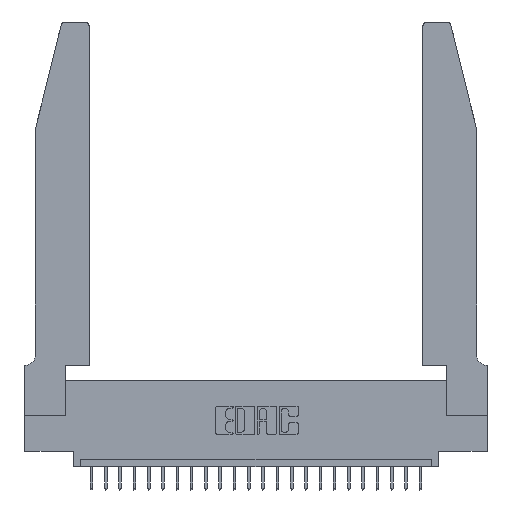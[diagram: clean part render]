
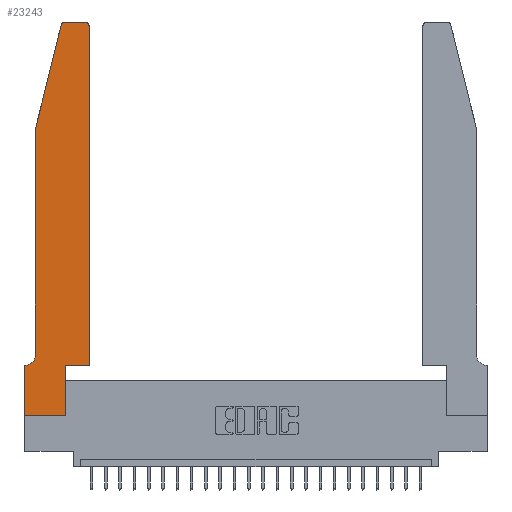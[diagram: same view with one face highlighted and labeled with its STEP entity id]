
A CAD part, top view. The second image highlights one B-rep face of the part: STEP entity #23243.
In plain terms, the highlighted planar face has unit normal (0, 0, 1).
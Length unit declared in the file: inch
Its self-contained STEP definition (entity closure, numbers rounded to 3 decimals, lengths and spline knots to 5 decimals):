
#17 = VERTEX_POINT ( 'NONE', #1038 ) ;
#164 = CARTESIAN_POINT ( 'NONE',  ( 0., 0.35, 0.37 ) ) ;
#499 = VERTEX_POINT ( 'NONE', #9481 ) ;
#1038 = CARTESIAN_POINT ( 'NONE',  ( 0., 0.35, 0.37 ) ) ;
#1136 = CIRCLE ( 'NONE', #16372, 0.03 ) ;
#1219 = DIRECTION ( 'NONE',  ( 1., 0., 0. ) ) ;
#1333 = ORIENTED_EDGE ( 'NONE', *, *, #2403, .T. ) ;
#1780 = EDGE_CURVE ( 'NONE', #19291, #17657, #18581, .T. ) ;
#1923 = VECTOR ( 'NONE', #10608, 39.37008 ) ;
#2403 = EDGE_CURVE ( 'NONE', #499, #18775, #5967, .T. ) ;
#2966 = EDGE_CURVE ( 'NONE', #12963, #6770, #20093, .T. ) ;
#3355 = DIRECTION ( 'NONE',  ( 0., 1., 0. ) ) ;
#3795 = CARTESIAN_POINT ( 'NONE',  ( 0.4205, 2.72, 0.37 ) ) ;
#3904 = DIRECTION ( 'NONE',  ( 0., 0., 1. ) ) ;
#4003 = CARTESIAN_POINT ( 'NONE',  ( 0.2865, 0.35, 0.37 ) ) ;
#4143 = ORIENTED_EDGE ( 'NONE', *, *, #11249, .T. ) ;
#4719 = ORIENTED_EDGE ( 'NONE', *, *, #18608, .T. ) ;
#4771 = EDGE_CURVE ( 'NONE', #24978, #9775, #20688, .T. ) ;
#4891 = DIRECTION ( 'NONE',  ( 0., -1., 0. ) ) ;
#5760 = CARTESIAN_POINT ( 'NONE',  ( 0.0755, 2., 0.37 ) ) ;
#5800 = ORIENTED_EDGE ( 'NONE', *, *, #8507, .T. ) ;
#5967 = LINE ( 'NONE', #8858, #24112 ) ;
#6113 = VECTOR ( 'NONE', #22655, 39.37008 ) ;
#6178 = PLANE ( 'NONE',  #9769 ) ;
#6311 = DIRECTION ( 'NONE',  ( 0., 1., 0. ) ) ;
#6721 = LINE ( 'NONE', #14429, #15346 ) ;
#6731 = EDGE_CURVE ( 'NONE', #17, #19291, #6721, .T. ) ;
#6770 = VERTEX_POINT ( 'NONE', #14850 ) ;
#6901 = CIRCLE ( 'NONE', #9035, 0.03 ) ;
#7571 = DIRECTION ( 'NONE',  ( 1., 0., 0. ) ) ;
#8059 = DIRECTION ( 'NONE',  ( 1., 0., 0. ) ) ;
#8093 = ORIENTED_EDGE ( 'NONE', *, *, #2966, .T. ) ;
#8507 = EDGE_CURVE ( 'NONE', #18775, #20206, #1136, .T. ) ;
#8521 = DIRECTION ( 'NONE',  ( 0., 0., -1. ) ) ;
#8858 = CARTESIAN_POINT ( 'NONE',  ( 0.2605, 2.75, 0.37 ) ) ;
#9035 = AXIS2_PLACEMENT_3D ( 'NONE', #3795, #17533, #7571 ) ;
#9481 = CARTESIAN_POINT ( 'NONE',  ( 0.4205, 2.75, 0.37 ) ) ;
#9558 = CARTESIAN_POINT ( 'NONE',  ( 0.284, 2.75, 0.37 ) ) ;
#9697 = CARTESIAN_POINT ( 'NONE',  ( 0.0055, 0.35, 0.37 ) ) ;
#9769 = AXIS2_PLACEMENT_3D ( 'NONE', #164, #17849, #8059 ) ;
#9775 = VERTEX_POINT ( 'NONE', #10046 ) ;
#10046 = CARTESIAN_POINT ( 'NONE',  ( 0.0755, 0.42, 0.37 ) ) ;
#10608 = DIRECTION ( 'NONE',  ( 0., -1., 0. ) ) ;
#11009 = AXIS2_PLACEMENT_3D ( 'NONE', #12983, #8521, #24862 ) ;
#11036 = ORIENTED_EDGE ( 'NONE', *, *, #1780, .T. ) ;
#11249 = EDGE_CURVE ( 'NONE', #23093, #17, #13479, .T. ) ;
#11271 = CARTESIAN_POINT ( 'NONE',  ( 0.0755, 2., 0.37 ) ) ;
#12072 = CARTESIAN_POINT ( 'NONE',  ( 0.0755, 2., 0.37 ) ) ;
#12230 = CARTESIAN_POINT ( 'NONE',  ( 0.2865, 0.35, 0.37 ) ) ;
#12297 = DIRECTION ( 'NONE',  ( 1., 0., 0. ) ) ;
#12811 = EDGE_CURVE ( 'NONE', #20206, #24978, #21098, .T. ) ;
#12849 = LINE ( 'NONE', #24775, #17482 ) ;
#12963 = VERTEX_POINT ( 'NONE', #17188 ) ;
#12983 = CARTESIAN_POINT ( 'NONE',  ( 0.0055, 0.42, 0.37 ) ) ;
#13020 = EDGE_CURVE ( 'NONE', #6770, #499, #6901, .T. ) ;
#13479 = LINE ( 'NONE', #20775, #6113 ) ;
#14429 = CARTESIAN_POINT ( 'NONE',  ( 0., 0., 0.37 ) ) ;
#14733 = ORIENTED_EDGE ( 'NONE', *, *, #18575, .T. ) ;
#14850 = CARTESIAN_POINT ( 'NONE',  ( 0.4505, 2.72, 0.37 ) ) ;
#14874 = VECTOR ( 'NONE', #3355, 39.37008 ) ;
#15112 = CARTESIAN_POINT ( 'NONE',  ( 0.4505, 0.35, 0.37 ) ) ;
#15346 = VECTOR ( 'NONE', #4891, 39.37008 ) ;
#15596 = CARTESIAN_POINT ( 'NONE',  ( 0.25487, 2.72718, 0.37 ) ) ;
#15671 = CARTESIAN_POINT ( 'NONE',  ( 0.284, 2.72, 0.37 ) ) ;
#16302 = FACE_OUTER_BOUND ( 'NONE', #22569, .T. ) ;
#16372 = AXIS2_PLACEMENT_3D ( 'NONE', #15671, #3904, #12297 ) ;
#17188 = CARTESIAN_POINT ( 'NONE',  ( 0.4505, 0.35, 0.37 ) ) ;
#17377 = VECTOR ( 'NONE', #19558, 39.37008 ) ;
#17482 = VECTOR ( 'NONE', #1219, 39.37008 ) ;
#17533 = DIRECTION ( 'NONE',  ( 0., 0., 1. ) ) ;
#17572 = CARTESIAN_POINT ( 'NONE',  ( 0., 0., 0.37 ) ) ;
#17657 = VERTEX_POINT ( 'NONE', #17917 ) ;
#17849 = DIRECTION ( 'NONE',  ( 0., 0., 1. ) ) ;
#17917 = CARTESIAN_POINT ( 'NONE',  ( 0.2865, 0., 0.37 ) ) ;
#18238 = DIRECTION ( 'NONE',  ( -0.239, -0.971, 0. ) ) ;
#18575 = EDGE_CURVE ( 'NONE', #9775, #23093, #22707, .T. ) ;
#18581 = LINE ( 'NONE', #17572, #17377 ) ;
#18608 = EDGE_CURVE ( 'NONE', #23737, #12963, #12849, .T. ) ;
#18775 = VERTEX_POINT ( 'NONE', #9558 ) ;
#19291 = VERTEX_POINT ( 'NONE', #23521 ) ;
#19558 = DIRECTION ( 'NONE',  ( 1., 0., 0. ) ) ;
#20093 = LINE ( 'NONE', #15112, #14874 ) ;
#20206 = VERTEX_POINT ( 'NONE', #15596 ) ;
#20315 = EDGE_CURVE ( 'NONE', #17657, #23737, #22605, .T. ) ;
#20688 = LINE ( 'NONE', #12072, #1923 ) ;
#20775 = CARTESIAN_POINT ( 'NONE',  ( 0.0755, 0.35, 0.37 ) ) ;
#20993 = ORIENTED_EDGE ( 'NONE', *, *, #12811, .T. ) ;
#21098 = LINE ( 'NONE', #11271, #23557 ) ;
#21930 = ORIENTED_EDGE ( 'NONE', *, *, #4771, .T. ) ;
#22522 = ORIENTED_EDGE ( 'NONE', *, *, #6731, .T. ) ;
#22569 = EDGE_LOOP ( 'NONE', ( #1333, #5800, #20993, #21930, #14733, #4143, #22522, #11036, #24105, #4719, #8093, #23311 ) ) ;
#22581 = VECTOR ( 'NONE', #6311, 39.37008 ) ;
#22605 = LINE ( 'NONE', #12230, #22581 ) ;
#22655 = DIRECTION ( 'NONE',  ( -1., 0., 0. ) ) ;
#22707 = CIRCLE ( 'NONE', #11009, 0.07 ) ;
#23093 = VERTEX_POINT ( 'NONE', #9697 ) ;
#23243 = ADVANCED_FACE ( 'NONE', ( #16302 ), #6178, .T. ) ;
#23311 = ORIENTED_EDGE ( 'NONE', *, *, #13020, .T. ) ;
#23521 = CARTESIAN_POINT ( 'NONE',  ( 0., 0., 0.37 ) ) ;
#23557 = VECTOR ( 'NONE', #18238, 39.37008 ) ;
#23737 = VERTEX_POINT ( 'NONE', #4003 ) ;
#24105 = ORIENTED_EDGE ( 'NONE', *, *, #20315, .T. ) ;
#24112 = VECTOR ( 'NONE', #24184, 39.37008 ) ;
#24184 = DIRECTION ( 'NONE',  ( -1., 0., 0. ) ) ;
#24775 = CARTESIAN_POINT ( 'NONE',  ( 0.4505, 0.35, 0.37 ) ) ;
#24862 = DIRECTION ( 'NONE',  ( -1., 0., 0. ) ) ;
#24978 = VERTEX_POINT ( 'NONE', #5760 ) ;
